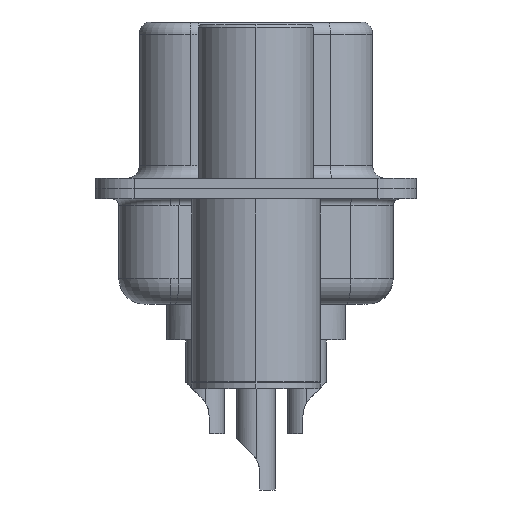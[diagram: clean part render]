
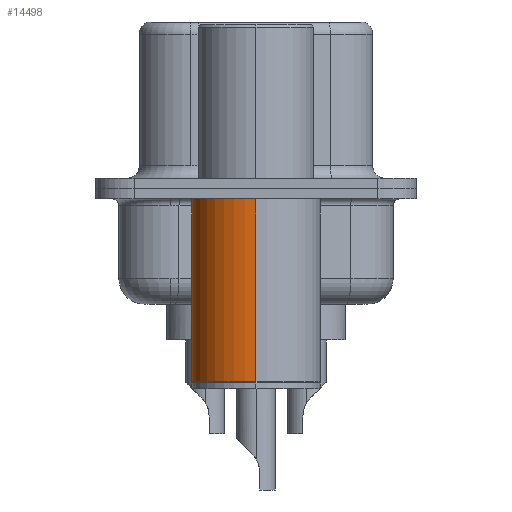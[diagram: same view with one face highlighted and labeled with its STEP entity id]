
A CAD part, left-side view. The second image highlights one B-rep face of the part: STEP entity #14498.
In plain terms, the highlighted cylindrical face has radius 2.5 mm (diameter 5 mm), a partial arc.
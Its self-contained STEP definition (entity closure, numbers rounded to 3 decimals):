
#103 = EDGE_CURVE ( 'NONE', #15723, #9470, #12102, .T. ) ;
#804 = DIRECTION ( 'NONE',  ( 0., 0., 1. ) ) ;
#1123 = ORIENTED_EDGE ( 'NONE', *, *, #17771, .T. ) ;
#1148 = AXIS2_PLACEMENT_3D ( 'NONE', #15600, #17369, #3248 ) ;
#1321 = DIRECTION ( 'NONE',  ( 1., 0., 0. ) ) ;
#1385 = CARTESIAN_POINT ( 'NONE',  ( 0., 0., -0.4 ) ) ;
#1397 = CARTESIAN_POINT ( 'NONE',  ( 2.5, 0., -7.525 ) ) ;
#2323 = DIRECTION ( 'NONE',  ( 1., 0., 0. ) ) ;
#2430 = DIRECTION ( 'NONE',  ( 0., 0., 1. ) ) ;
#2503 = CARTESIAN_POINT ( 'NONE',  ( 0., 0., -7.525 ) ) ;
#3120 = CIRCLE ( 'NONE', #21860, 2.5 ) ;
#3248 = DIRECTION ( 'NONE',  ( 1., 0., 0. ) ) ;
#4297 = EDGE_CURVE ( 'NONE', #8630, #13329, #3120, .T. ) ;
#5517 = ORIENTED_EDGE ( 'NONE', *, *, #7272, .F. ) ;
#6008 = CYLINDRICAL_SURFACE ( 'NONE', #1148, 2.5 ) ;
#7272 = EDGE_CURVE ( 'NONE', #15723, #8630, #12871, .T. ) ;
#7768 = LINE ( 'NONE', #13457, #20107 ) ;
#8630 = VERTEX_POINT ( 'NONE', #19785 ) ;
#8763 = VECTOR ( 'NONE', #21015, 1000. ) ;
#9470 = VERTEX_POINT ( 'NONE', #22349 ) ;
#10469 = CARTESIAN_POINT ( 'NONE',  ( 2.5, 0., 0.581 ) ) ;
#12102 = CIRCLE ( 'NONE', #21638, 2.5 ) ;
#12871 = LINE ( 'NONE', #10469, #8763 ) ;
#13329 = VERTEX_POINT ( 'NONE', #16268 ) ;
#13457 = CARTESIAN_POINT ( 'NONE',  ( -2.5, 0., 0.581 ) ) ;
#14498 = ADVANCED_FACE ( 'NONE', ( #20036 ), #6008, .T. ) ;
#15227 = DIRECTION ( 'NONE',  ( 0., 0., 1. ) ) ;
#15600 = CARTESIAN_POINT ( 'NONE',  ( 0., 0., 0.581 ) ) ;
#15723 = VERTEX_POINT ( 'NONE', #1397 ) ;
#16268 = CARTESIAN_POINT ( 'NONE',  ( -2.5, 0., -0.4 ) ) ;
#16350 = ORIENTED_EDGE ( 'NONE', *, *, #4297, .F. ) ;
#16785 = ORIENTED_EDGE ( 'NONE', *, *, #103, .T. ) ;
#17369 = DIRECTION ( 'NONE',  ( 0., 0., 1. ) ) ;
#17771 = EDGE_CURVE ( 'NONE', #9470, #13329, #7768, .T. ) ;
#19785 = CARTESIAN_POINT ( 'NONE',  ( 2.5, 0., -0.4 ) ) ;
#20036 = FACE_OUTER_BOUND ( 'NONE', #20316, .T. ) ;
#20107 = VECTOR ( 'NONE', #15227, 1000. ) ;
#20316 = EDGE_LOOP ( 'NONE', ( #16785, #1123, #16350, #5517 ) ) ;
#21015 = DIRECTION ( 'NONE',  ( 0., 0., 1. ) ) ;
#21638 = AXIS2_PLACEMENT_3D ( 'NONE', #2503, #2430, #2323 ) ;
#21860 = AXIS2_PLACEMENT_3D ( 'NONE', #1385, #804, #1321 ) ;
#22349 = CARTESIAN_POINT ( 'NONE',  ( -2.5, 0., -7.525 ) ) ;
